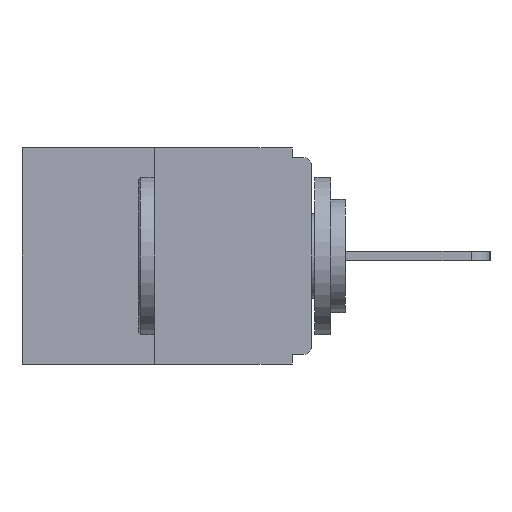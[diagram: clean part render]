
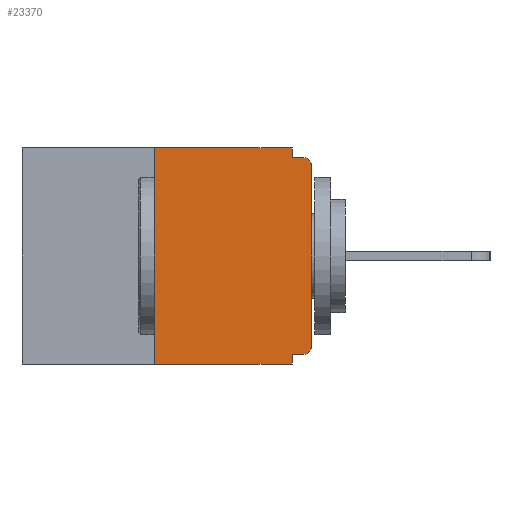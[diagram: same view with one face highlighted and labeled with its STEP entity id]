
A CAD part, left-side view. The second image highlights one B-rep face of the part: STEP entity #23370.
In plain terms, the highlighted planar face has unit normal (-1, 0, 0).
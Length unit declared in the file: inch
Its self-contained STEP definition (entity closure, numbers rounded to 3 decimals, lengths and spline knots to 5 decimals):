
#122 = CARTESIAN_POINT ( 'NONE',  ( 0., 0.015, -0.328 ) ) ;
#496 = LINE ( 'NONE', #11221, #11604 ) ;
#702 = ORIENTED_EDGE ( 'NONE', *, *, #12961, .F. ) ;
#1148 = CARTESIAN_POINT ( 'NONE',  ( 0., 0., -0.03 ) ) ;
#1177 = VERTEX_POINT ( 'NONE', #9537 ) ;
#1298 = VERTEX_POINT ( 'NONE', #12589 ) ;
#2033 = DIRECTION ( 'NONE',  ( 0., 0., -1. ) ) ;
#2131 = EDGE_CURVE ( 'NONE', #9561, #14679, #9069, .T. ) ;
#2477 = AXIS2_PLACEMENT_3D ( 'NONE', #5429, #7225, #5215 ) ;
#3612 = AXIS2_PLACEMENT_3D ( 'NONE', #20874, #4556, #8214 ) ;
#4164 = EDGE_CURVE ( 'NONE', #14679, #1177, #496, .T. ) ;
#4462 = VECTOR ( 'NONE', #17364, 39.37008 ) ;
#4556 = DIRECTION ( 'NONE',  ( 1., 0., 0. ) ) ;
#4656 = LINE ( 'NONE', #10005, #16149 ) ;
#4777 = CARTESIAN_POINT ( 'NONE',  ( 0., 0.25, 0. ) ) ;
#4952 = CARTESIAN_POINT ( 'NONE',  ( 0., 0.25, 0. ) ) ;
#5147 = DIRECTION ( 'NONE',  ( 0., 0., -1. ) ) ;
#5215 = DIRECTION ( 'NONE',  ( 0., 0., -1. ) ) ;
#5429 = CARTESIAN_POINT ( 'NONE',  ( 0., 0.015, -0.03 ) ) ;
#5442 = VECTOR ( 'NONE', #10525, 39.37008 ) ;
#5725 = LINE ( 'NONE', #20744, #17305 ) ;
#6122 = VERTEX_POINT ( 'NONE', #14792 ) ;
#7223 = ORIENTED_EDGE ( 'NONE', *, *, #23246, .F. ) ;
#7225 = DIRECTION ( 'NONE',  ( -1., 0., 0. ) ) ;
#7526 = EDGE_LOOP ( 'NONE', ( #21626, #21496, #22439, #702, #7223, #12902, #10789, #9420, #18347, #19305 ) ) ;
#8214 = DIRECTION ( 'NONE',  ( 0., 0., -1. ) ) ;
#8467 = CARTESIAN_POINT ( 'NONE',  ( 0., 0.015, -0.313 ) ) ;
#8570 = VERTEX_POINT ( 'NONE', #17254 ) ;
#8811 = EDGE_CURVE ( 'NONE', #17199, #8570, #17681, .T. ) ;
#9059 = EDGE_CURVE ( 'NONE', #18337, #18230, #17331, .T. ) ;
#9069 = LINE ( 'NONE', #16072, #14769 ) ;
#9420 = ORIENTED_EDGE ( 'NONE', *, *, #8811, .T. ) ;
#9526 = CARTESIAN_POINT ( 'NONE',  ( 0., 0.031, 0. ) ) ;
#9537 = CARTESIAN_POINT ( 'NONE',  ( 0., 0.031, -0.015 ) ) ;
#9561 = VERTEX_POINT ( 'NONE', #4777 ) ;
#10005 = CARTESIAN_POINT ( 'NONE',  ( 0., 0., -0.328 ) ) ;
#10080 = LINE ( 'NONE', #4952, #4462 ) ;
#10525 = DIRECTION ( 'NONE',  ( 0., 0., 1. ) ) ;
#10789 = ORIENTED_EDGE ( 'NONE', *, *, #17757, .T. ) ;
#11221 = CARTESIAN_POINT ( 'NONE',  ( 0., 0.031, 0. ) ) ;
#11498 = EDGE_CURVE ( 'NONE', #1177, #8570, #23498, .T. ) ;
#11604 = VECTOR ( 'NONE', #2033, 39.37008 ) ;
#11925 = DIRECTION ( 'NONE',  ( 0., 1., 0. ) ) ;
#12185 = CARTESIAN_POINT ( 'NONE',  ( 0., 0., -0.313 ) ) ;
#12317 = LINE ( 'NONE', #19583, #5442 ) ;
#12589 = CARTESIAN_POINT ( 'NONE',  ( 0., 0.031, -0.328 ) ) ;
#12785 = EDGE_CURVE ( 'NONE', #19061, #9561, #10080, .T. ) ;
#12902 = ORIENTED_EDGE ( 'NONE', *, *, #9059, .T. ) ;
#12961 = EDGE_CURVE ( 'NONE', #1298, #6122, #20317, .T. ) ;
#14636 = CARTESIAN_POINT ( 'NONE',  ( 0., 0.25, -0.343 ) ) ;
#14679 = VERTEX_POINT ( 'NONE', #9526 ) ;
#14769 = VECTOR ( 'NONE', #18251, 39.37008 ) ;
#14792 = CARTESIAN_POINT ( 'NONE',  ( 0., 0.031, -0.343 ) ) ;
#15043 = VECTOR ( 'NONE', #19819, 39.37008 ) ;
#15163 = DIRECTION ( 'NONE',  ( 0., -1., 0. ) ) ;
#15840 = FACE_OUTER_BOUND ( 'NONE', #7526, .T. ) ;
#16072 = CARTESIAN_POINT ( 'NONE',  ( 0., 0.46, 0. ) ) ;
#16149 = VECTOR ( 'NONE', #11925, 39.37008 ) ;
#16564 = AXIS2_PLACEMENT_3D ( 'NONE', #8467, #23359, #5147 ) ;
#17014 = VECTOR ( 'NONE', #22104, 39.37008 ) ;
#17199 = VERTEX_POINT ( 'NONE', #1148 ) ;
#17254 = CARTESIAN_POINT ( 'NONE',  ( 0., 0.015, -0.015 ) ) ;
#17305 = VECTOR ( 'NONE', #15163, 39.37008 ) ;
#17331 = CIRCLE ( 'NONE', #16564, 0.015 ) ;
#17364 = DIRECTION ( 'NONE',  ( 0., 0., 1. ) ) ;
#17681 = CIRCLE ( 'NONE', #2477, 0.015 ) ;
#17757 = EDGE_CURVE ( 'NONE', #18230, #17199, #12317, .T. ) ;
#17910 = CARTESIAN_POINT ( 'NONE',  ( 0., 0., -0.015 ) ) ;
#18230 = VERTEX_POINT ( 'NONE', #12185 ) ;
#18251 = DIRECTION ( 'NONE',  ( 0., -1., 0. ) ) ;
#18337 = VERTEX_POINT ( 'NONE', #122 ) ;
#18347 = ORIENTED_EDGE ( 'NONE', *, *, #11498, .F. ) ;
#18552 = CARTESIAN_POINT ( 'NONE',  ( 0., 0.031, -0.343 ) ) ;
#19061 = VERTEX_POINT ( 'NONE', #14636 ) ;
#19305 = ORIENTED_EDGE ( 'NONE', *, *, #4164, .F. ) ;
#19583 = CARTESIAN_POINT ( 'NONE',  ( 0., 0., 0. ) ) ;
#19819 = DIRECTION ( 'NONE',  ( 0., -1., 0. ) ) ;
#20317 = LINE ( 'NONE', #18552, #17014 ) ;
#20744 = CARTESIAN_POINT ( 'NONE',  ( 0., 0.46, -0.343 ) ) ;
#20874 = CARTESIAN_POINT ( 'NONE',  ( 0., 0.46, 0. ) ) ;
#21324 = PLANE ( 'NONE',  #3612 ) ;
#21496 = ORIENTED_EDGE ( 'NONE', *, *, #12785, .F. ) ;
#21626 = ORIENTED_EDGE ( 'NONE', *, *, #2131, .F. ) ;
#22104 = DIRECTION ( 'NONE',  ( 0., 0., -1. ) ) ;
#22439 = ORIENTED_EDGE ( 'NONE', *, *, #23195, .T. ) ;
#23195 = EDGE_CURVE ( 'NONE', #19061, #6122, #5725, .T. ) ;
#23246 = EDGE_CURVE ( 'NONE', #18337, #1298, #4656, .T. ) ;
#23359 = DIRECTION ( 'NONE',  ( -1., 0., 0. ) ) ;
#23370 = ADVANCED_FACE ( 'NONE', ( #15840 ), #21324, .F. ) ;
#23498 = LINE ( 'NONE', #17910, #15043 ) ;
